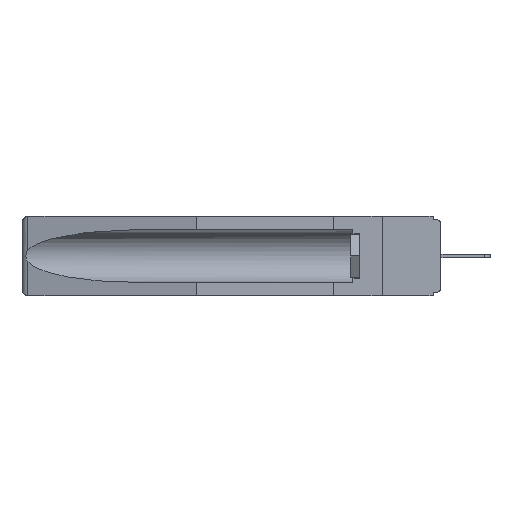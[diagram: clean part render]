
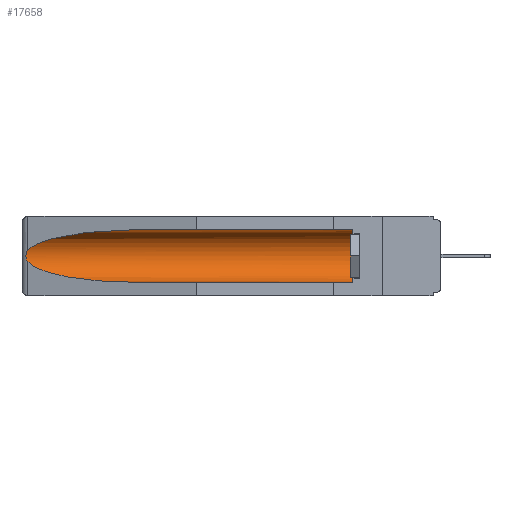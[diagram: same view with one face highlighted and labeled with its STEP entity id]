
A CAD part, left-side view. The second image highlights one B-rep face of the part: STEP entity #17658.
In plain terms, the highlighted cylindrical face has radius 2.857 mm (diameter 5.715 mm), a partial arc.
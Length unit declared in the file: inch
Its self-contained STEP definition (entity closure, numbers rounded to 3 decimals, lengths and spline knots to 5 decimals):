
#111 = CARTESIAN_POINT ( 'NONE',  ( 0.26537, 1.52718, -0.19328 ) ) ;
#201 = CYLINDRICAL_SURFACE ( 'NONE', #14134, 0.1125 ) ;
#568 =( BOUNDED_CURVE ( )  B_SPLINE_CURVE ( 3, ( #4269, #2850, #14662, #5817 ),
 .UNSPECIFIED., .F., .T. ) 
 B_SPLINE_CURVE_WITH_KNOTS ( ( 4, 4 ),
 ( 4.71239, 6.08839 ),
 .UNSPECIFIED. ) 
 CURVE ( )  GEOMETRIC_REPRESENTATION_ITEM ( )  RATIONAL_B_SPLINE_CURVE ( ( 1., 0.848, 0.848, 1. ) ) 
 REPRESENTATION_ITEM ( '' )  );
#808 = CARTESIAN_POINT ( 'NONE',  ( 0.2673, 1.5327, -0.16383 ) ) ;
#853 = CARTESIAN_POINT ( 'NONE',  ( 0.26537, 1.52718, -0.14972 ) ) ;
#1035 = EDGE_CURVE ( 'NONE', #6470, #11455, #14742, .T. ) ;
#1301 = DIRECTION ( 'NONE',  ( 0., 0., 1. ) ) ;
#2116 = AXIS2_PLACEMENT_3D ( 'NONE', #5435, #15766, #6922 ) ;
#2850 = CARTESIAN_POINT ( 'NONE',  ( 0.21114, 1.30732, -0.059 ) ) ;
#3407 = VERTEX_POINT ( 'NONE', #6370 ) ;
#3423 = CARTESIAN_POINT ( 'NONE',  ( 0.26537, 1.52718, -0.19328 ) ) ;
#3614 = CARTESIAN_POINT ( 'NONE',  ( 0.155, 1.07973, -0.284 ) ) ;
#3657 = EDGE_CURVE ( 'NONE', #10075, #15934, #6188, .T. ) ;
#3762 = ORIENTED_EDGE ( 'NONE', *, *, #9246, .T. ) ;
#4269 = CARTESIAN_POINT ( 'NONE',  ( 0.155, 1.07973, -0.059 ) ) ;
#4630 = DIRECTION ( 'NONE',  ( 0., 1., 0. ) ) ;
#5023 = CARTESIAN_POINT ( 'NONE',  ( 0.155, 0.126, -0.284 ) ) ;
#5364 = ORIENTED_EDGE ( 'NONE', *, *, #14265, .T. ) ;
#5435 = CARTESIAN_POINT ( 'NONE',  ( 0.155, 0.126, -0.1715 ) ) ;
#5607 = CARTESIAN_POINT ( 'NONE',  ( 0.26655, 1.53094, -0.18657 ) ) ;
#5817 = CARTESIAN_POINT ( 'NONE',  ( 0.26537, 1.52718, -0.14972 ) ) ;
#5924 = CARTESIAN_POINT ( 'NONE',  ( 0.155, 0.126, -0.059 ) ) ;
#6188 = B_SPLINE_CURVE_WITH_KNOTS ( 'NONE', 3,
 ( #853, #7794, #18775, #808, #18834, #18791, #18737, #5607, #18301, #18257 ),
 .UNSPECIFIED., .F., .F.,
 ( 4, 2, 2, 2, 4 ),
 ( 0., 0.00029, 0.00058, 0.00087, 0.00117 ),
 .UNSPECIFIED. ) ;
#6364 = CARTESIAN_POINT ( 'NONE',  ( 0.21114, 1.30732, -0.284 ) ) ;
#6370 = CARTESIAN_POINT ( 'NONE',  ( 0.155, 1.07973, -0.059 ) ) ;
#6470 = VERTEX_POINT ( 'NONE', #5023 ) ;
#6879 = VECTOR ( 'NONE', #4630, 39.37008 ) ;
#6922 = DIRECTION ( 'NONE',  ( 0., 0., 1. ) ) ;
#7349 = LINE ( 'NONE', #7572, #6879 ) ;
#7572 = CARTESIAN_POINT ( 'NONE',  ( 0.155, -0.30754, -0.059 ) ) ;
#7651 = ORIENTED_EDGE ( 'NONE', *, *, #13182, .T. ) ;
#7794 = CARTESIAN_POINT ( 'NONE',  ( 0.26597, 1.52961, -0.15275 ) ) ;
#8425 = FACE_OUTER_BOUND ( 'NONE', #15809, .T. ) ;
#8913 = EDGE_CURVE ( 'NONE', #15930, #3407, #7349, .T. ) ;
#9246 = EDGE_CURVE ( 'NONE', #6470, #15930, #9628, .T. ) ;
#9628 = CIRCLE ( 'NONE', #2116, 0.1125 ) ;
#10075 = VERTEX_POINT ( 'NONE', #14892 ) ;
#11455 = VERTEX_POINT ( 'NONE', #3614 ) ;
#11522 = ORIENTED_EDGE ( 'NONE', *, *, #3657, .T. ) ;
#11559 = CARTESIAN_POINT ( 'NONE',  ( 0.155, -0.30754, -0.1715 ) ) ;
#11698 = VECTOR ( 'NONE', #18771, 39.37008 ) ;
#11780 = ORIENTED_EDGE ( 'NONE', *, *, #8913, .T. ) ;
#12226 = CARTESIAN_POINT ( 'NONE',  ( 0.25451, 1.48313, -0.24835 ) ) ;
#13157 = ORIENTED_EDGE ( 'NONE', *, *, #1035, .F. ) ;
#13182 = EDGE_CURVE ( 'NONE', #15934, #11455, #14236, .T. ) ;
#13284 = CARTESIAN_POINT ( 'NONE',  ( 0.155, -0.30754, -0.284 ) ) ;
#14134 = AXIS2_PLACEMENT_3D ( 'NONE', #11559, #18980, #1301 ) ;
#14236 =( BOUNDED_CURVE ( )  B_SPLINE_CURVE ( 3, ( #3423, #12226, #6364, #16722 ),
 .UNSPECIFIED., .F., .T. ) 
 B_SPLINE_CURVE_WITH_KNOTS ( ( 4, 4 ),
 ( 0.1948, 1.5708 ),
 .UNSPECIFIED. ) 
 CURVE ( )  GEOMETRIC_REPRESENTATION_ITEM ( )  RATIONAL_B_SPLINE_CURVE ( ( 1., 0.848, 0.848, 1. ) ) 
 REPRESENTATION_ITEM ( '' )  );
#14265 = EDGE_CURVE ( 'NONE', #3407, #10075, #568, .T. ) ;
#14662 = CARTESIAN_POINT ( 'NONE',  ( 0.25451, 1.48313, -0.09465 ) ) ;
#14742 = LINE ( 'NONE', #13284, #11698 ) ;
#14892 = CARTESIAN_POINT ( 'NONE',  ( 0.26537, 1.52718, -0.14972 ) ) ;
#15766 = DIRECTION ( 'NONE',  ( 0., -1., 0. ) ) ;
#15809 = EDGE_LOOP ( 'NONE', ( #5364, #11522, #7651, #13157, #3762, #11780 ) ) ;
#15930 = VERTEX_POINT ( 'NONE', #5924 ) ;
#15934 = VERTEX_POINT ( 'NONE', #111 ) ;
#16722 = CARTESIAN_POINT ( 'NONE',  ( 0.155, 1.07973, -0.284 ) ) ;
#17658 = ADVANCED_FACE ( 'NONE', ( #8425 ), #201, .F. ) ;
#18257 = CARTESIAN_POINT ( 'NONE',  ( 0.26537, 1.52718, -0.19328 ) ) ;
#18301 = CARTESIAN_POINT ( 'NONE',  ( 0.26597, 1.5296, -0.19026 ) ) ;
#18737 = CARTESIAN_POINT ( 'NONE',  ( 0.2673, 1.53269, -0.17917 ) ) ;
#18771 = DIRECTION ( 'NONE',  ( 0., 1., 0. ) ) ;
#18775 = CARTESIAN_POINT ( 'NONE',  ( 0.26654, 1.53092, -0.15636 ) ) ;
#18791 = CARTESIAN_POINT ( 'NONE',  ( 0.2675, 1.53308, -0.17534 ) ) ;
#18834 = CARTESIAN_POINT ( 'NONE',  ( 0.2675, 1.53308, -0.16763 ) ) ;
#18980 = DIRECTION ( 'NONE',  ( 0., 1., 0. ) ) ;
